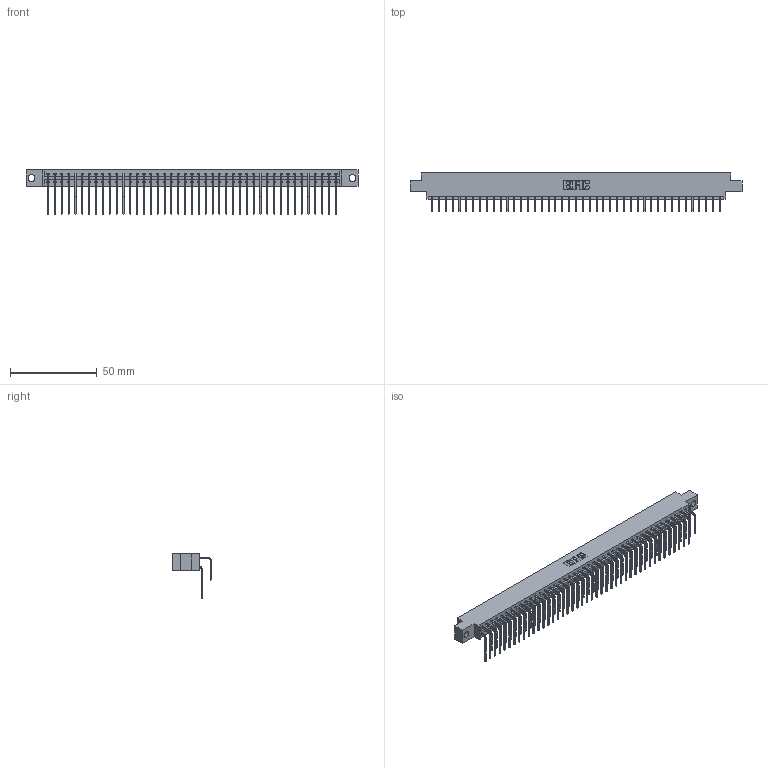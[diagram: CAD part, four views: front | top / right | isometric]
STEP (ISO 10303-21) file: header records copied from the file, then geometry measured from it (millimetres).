
FILE_DESCRIPTION (( 'STEP AP203' ), '1' );
FILE_NAME ('333-086-558-804.STEP', '2018-08-05T06:55:15', ( '' ), ( '' ), 'SwSTEP 2.0', 'SolidWorks 2016', '' );
FILE_SCHEMA (( 'CONFIG_CONTROL_DESIGN' ));
Length unit declared in the file: inch
Products named in the file (4): 333-086-558-804; 333 Part_Offset - .156 Dia - TH; 345-292-001_558 559 Tail - 1; 345-292-001_558 Tail - 2
Assembly tree (87 placements, depth 2):
  333-086-558-804
    333 Part_Offset - .156 Dia - TH
    345-292-001_558 559 Tail - 1  x43
    345-292-001_558 Tail - 2  x43
Bounding box: 191.92 x 22.17 x 25.53 mm (x, y, z)
Volume: 19784 mm3; surface area: 25891.8 mm2
Topology: 87 solids, 87 shells, 4762 faces, 14169 edges, 9330 vertices
Faces by surface type: plane 3342, cylinder 1420
Entity records: 29453 total; most frequent: CARTESIAN_POINT 4933, ORIENTED_EDGE 4818, DIRECTION 4193, EDGE_CURVE 2409, VECTOR 2241, LINE 2241, VERTEX_POINT 1602, AXIS2_PLACEMENT_3D 976
